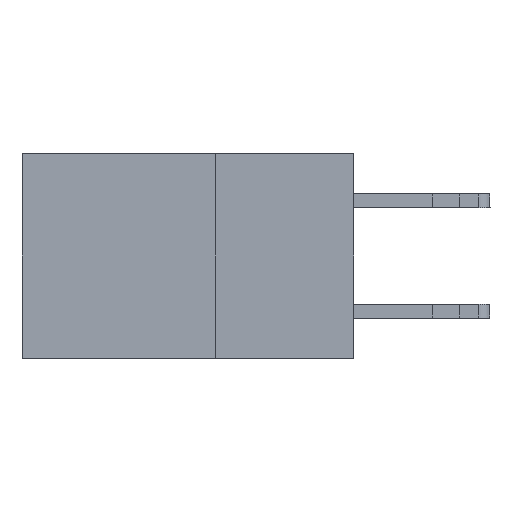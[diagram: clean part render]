
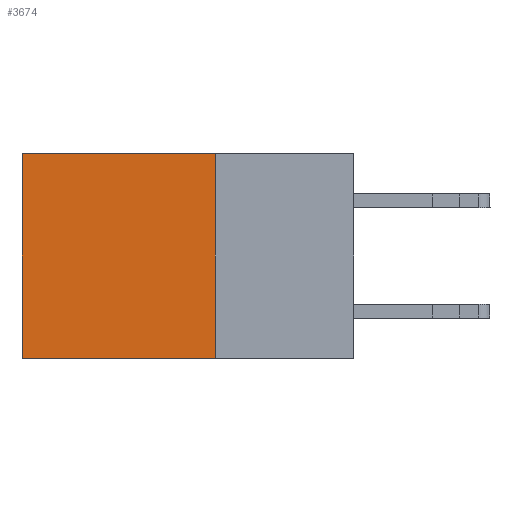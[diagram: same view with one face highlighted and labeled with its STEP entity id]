
A CAD part, left-side view. The second image highlights one B-rep face of the part: STEP entity #3674.
In plain terms, the highlighted planar face has unit normal (-1, 0, 0).
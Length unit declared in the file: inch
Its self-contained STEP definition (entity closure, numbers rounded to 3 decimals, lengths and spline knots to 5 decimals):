
#779 = ORIENTED_EDGE ( 'NONE', *, *, #4446, .T. ) ;
#798 = LINE ( 'NONE', #13145, #11179 ) ;
#1526 = VECTOR ( 'NONE', #2489, 39.37008 ) ;
#2489 = DIRECTION ( 'NONE',  ( 0., 1., 0. ) ) ;
#2866 = CARTESIAN_POINT ( 'NONE',  ( 0.2875, 0.6, -0.37 ) ) ;
#3674 = ADVANCED_FACE ( 'NONE', ( #6880 ), #16647, .F. ) ;
#3750 = CARTESIAN_POINT ( 'NONE',  ( 0.2875, 0.25, 0. ) ) ;
#4167 = CARTESIAN_POINT ( 'NONE',  ( 0.2875, 0.25, 0. ) ) ;
#4307 = CARTESIAN_POINT ( 'NONE',  ( 0.2875, 0.6, 0. ) ) ;
#4414 = CARTESIAN_POINT ( 'NONE',  ( 0.2875, 0.25, 0. ) ) ;
#4446 = EDGE_CURVE ( 'NONE', #5475, #8331, #7541, .T. ) ;
#5264 = AXIS2_PLACEMENT_3D ( 'NONE', #4167, #15897, #11691 ) ;
#5475 = VERTEX_POINT ( 'NONE', #4414 ) ;
#6117 = DIRECTION ( 'NONE',  ( 0., 1., 0. ) ) ;
#6194 = CARTESIAN_POINT ( 'NONE',  ( 0.2875, 0.25, 0. ) ) ;
#6244 = EDGE_CURVE ( 'NONE', #5475, #6285, #17581, .T. ) ;
#6285 = VERTEX_POINT ( 'NONE', #13744 ) ;
#6880 = FACE_OUTER_BOUND ( 'NONE', #14709, .T. ) ;
#7541 = LINE ( 'NONE', #6194, #1526 ) ;
#7681 = CARTESIAN_POINT ( 'NONE',  ( 0.2875, 0.6, 0. ) ) ;
#8331 = VERTEX_POINT ( 'NONE', #7681 ) ;
#8373 = EDGE_CURVE ( 'NONE', #8331, #16985, #12168, .T. ) ;
#8569 = ORIENTED_EDGE ( 'NONE', *, *, #6244, .F. ) ;
#11179 = VECTOR ( 'NONE', #6117, 39.37008 ) ;
#11691 = DIRECTION ( 'NONE',  ( 0., 0., -1. ) ) ;
#12168 = LINE ( 'NONE', #4307, #17871 ) ;
#13145 = CARTESIAN_POINT ( 'NONE',  ( 0.2875, 0.25, -0.37 ) ) ;
#13712 = ORIENTED_EDGE ( 'NONE', *, *, #8373, .T. ) ;
#13744 = CARTESIAN_POINT ( 'NONE',  ( 0.2875, 0.25, -0.37 ) ) ;
#14709 = EDGE_LOOP ( 'NONE', ( #13712, #15526, #8569, #779 ) ) ;
#14858 = DIRECTION ( 'NONE',  ( 0., 0., -1. ) ) ;
#15093 = DIRECTION ( 'NONE',  ( 0., 0., -1. ) ) ;
#15526 = ORIENTED_EDGE ( 'NONE', *, *, #15811, .F. ) ;
#15811 = EDGE_CURVE ( 'NONE', #6285, #16985, #798, .T. ) ;
#15897 = DIRECTION ( 'NONE',  ( 1., 0., 0. ) ) ;
#16647 = PLANE ( 'NONE',  #5264 ) ;
#16985 = VERTEX_POINT ( 'NONE', #2866 ) ;
#17211 = VECTOR ( 'NONE', #14858, 39.37008 ) ;
#17581 = LINE ( 'NONE', #3750, #17211 ) ;
#17871 = VECTOR ( 'NONE', #15093, 39.37008 ) ;
